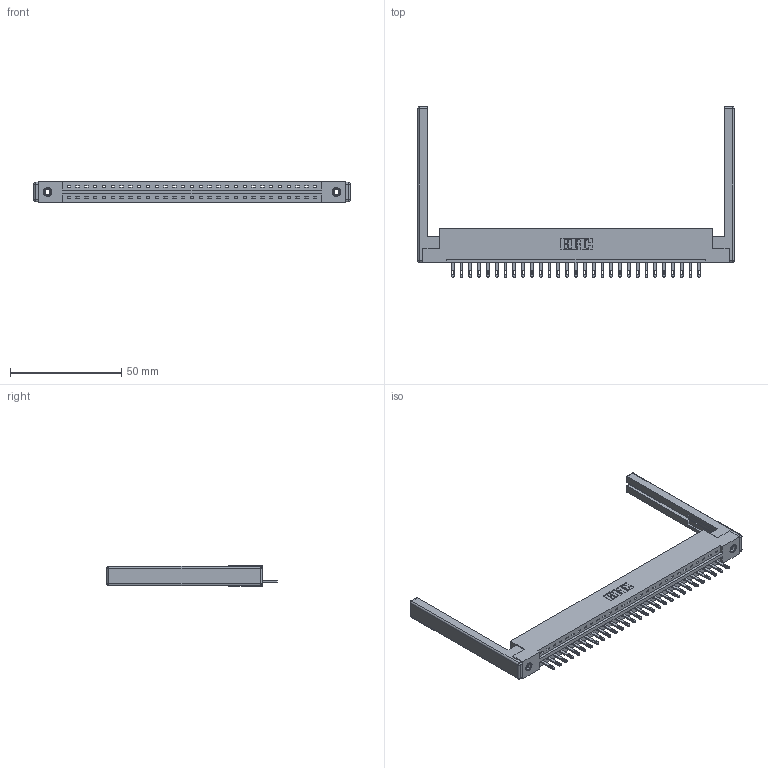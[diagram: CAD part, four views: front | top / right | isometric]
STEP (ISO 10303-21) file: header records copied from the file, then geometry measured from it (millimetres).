
FILE_DESCRIPTION (( 'STEP AP203' ), '1' );
FILE_NAME ('337-029-500-168.STEP', '2019-09-30T21:42:46', ( '' ), ( '' ), 'SwSTEP 2.0', 'SolidWorks 2016', '' );
FILE_SCHEMA (( 'CONFIG_CONTROL_DESIGN' ));
Length unit declared in the file: inch
Products named in the file (5): 307-220-068; 345-292-001_345-293-100; 337-029-500-168; 337 Part_Flush Mounting Lugs - 0.156 Dia-TI; 345-250-001_345-250-001-102
Assembly tree (34 placements, depth 2):
  337-029-500-168
    337 Part_Flush Mounting Lugs - 0.156 Dia-TI
    345-292-001_345-293-100  x29
    345-250-001_345-250-001-102  x2
    307-220-068  x2
Bounding box: 142.34 x 76.59 x 9.4 mm (x, y, z)
Volume: 19040.5 mm3; surface area: 19226.1 mm2
Topology: 34 solids, 34 shells, 1950 faces, 5921 edges, 3926 vertices
Faces by surface type: plane 1318, cylinder 608, cone 12, sphere 8, torus 4
Entity records: 25928 total; most frequent: CARTESIAN_POINT 4470, ORIENTED_EDGE 4424, DIRECTION 3864, EDGE_CURVE 2212, LINE 2030, VECTOR 2030, VERTEX_POINT 1466, AXIS2_PLACEMENT_3D 917
